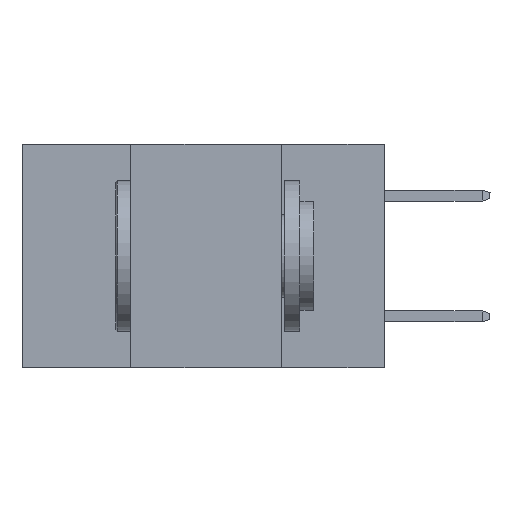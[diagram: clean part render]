
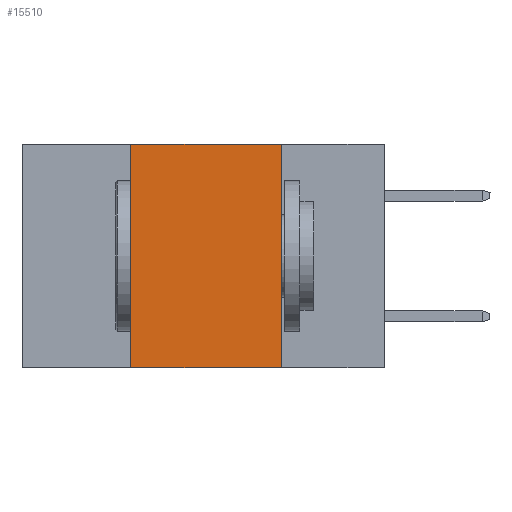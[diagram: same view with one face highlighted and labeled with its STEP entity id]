
A CAD part, left-side view. The second image highlights one B-rep face of the part: STEP entity #15510.
In plain terms, the highlighted planar face has unit normal (-1, 0, 0).
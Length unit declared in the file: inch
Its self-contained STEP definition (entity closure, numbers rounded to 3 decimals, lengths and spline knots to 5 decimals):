
#554 = CARTESIAN_POINT ( 'NONE',  ( 0., 0.42, -0.37 ) ) ;
#596 = CARTESIAN_POINT ( 'NONE',  ( 0., 0.17, 0. ) ) ;
#2267 = EDGE_CURVE ( 'NONE', #15436, #13225, #12381, .T. ) ;
#2889 = CARTESIAN_POINT ( 'NONE',  ( 0., 0.6, -0.37 ) ) ;
#3424 = FACE_OUTER_BOUND ( 'NONE', #23244, .T. ) ;
#3521 = EDGE_CURVE ( 'NONE', #15436, #8907, #11487, .T. ) ;
#3644 = DIRECTION ( 'NONE',  ( 1., 0., 0. ) ) ;
#3717 = DIRECTION ( 'NONE',  ( 0., 0., -1. ) ) ;
#4435 = EDGE_CURVE ( 'NONE', #13225, #18013, #20338, .T. ) ;
#5271 = CARTESIAN_POINT ( 'NONE',  ( 0., 0.42, 0. ) ) ;
#6875 = CARTESIAN_POINT ( 'NONE',  ( 0., 0.17, 0. ) ) ;
#7114 = DIRECTION ( 'NONE',  ( 0., 0., 1. ) ) ;
#7845 = CARTESIAN_POINT ( 'NONE',  ( 0., 0.6, 0. ) ) ;
#8907 = VERTEX_POINT ( 'NONE', #11901 ) ;
#9525 = DIRECTION ( 'NONE',  ( 0., -1., 0. ) ) ;
#9925 = EDGE_CURVE ( 'NONE', #18013, #8907, #14863, .T. ) ;
#10657 = VECTOR ( 'NONE', #7114, 39.37008 ) ;
#11014 = PLANE ( 'NONE',  #20922 ) ;
#11487 = LINE ( 'NONE', #2889, #20969 ) ;
#11901 = CARTESIAN_POINT ( 'NONE',  ( 0., 0.17, -0.37 ) ) ;
#12278 = VECTOR ( 'NONE', #18530, 39.37008 ) ;
#12381 = LINE ( 'NONE', #5271, #10657 ) ;
#13225 = VERTEX_POINT ( 'NONE', #22708 ) ;
#14863 = LINE ( 'NONE', #6875, #12278 ) ;
#15080 = ORIENTED_EDGE ( 'NONE', *, *, #9925, .F. ) ;
#15436 = VERTEX_POINT ( 'NONE', #554 ) ;
#15510 = ADVANCED_FACE ( 'NONE', ( #3424 ), #11014, .F. ) ;
#16098 = ORIENTED_EDGE ( 'NONE', *, *, #2267, .F. ) ;
#18013 = VERTEX_POINT ( 'NONE', #596 ) ;
#18530 = DIRECTION ( 'NONE',  ( 0., 0., -1. ) ) ;
#19478 = VECTOR ( 'NONE', #9525, 39.37008 ) ;
#19995 = ORIENTED_EDGE ( 'NONE', *, *, #4435, .F. ) ;
#20338 = LINE ( 'NONE', #7845, #19478 ) ;
#20922 = AXIS2_PLACEMENT_3D ( 'NONE', #21854, #3644, #3717 ) ;
#20969 = VECTOR ( 'NONE', #21330, 39.37008 ) ;
#21191 = ORIENTED_EDGE ( 'NONE', *, *, #3521, .T. ) ;
#21330 = DIRECTION ( 'NONE',  ( 0., -1., 0. ) ) ;
#21854 = CARTESIAN_POINT ( 'NONE',  ( 0., 0.6, 0. ) ) ;
#22708 = CARTESIAN_POINT ( 'NONE',  ( 0., 0.42, 0. ) ) ;
#23244 = EDGE_LOOP ( 'NONE', ( #15080, #19995, #16098, #21191 ) ) ;
